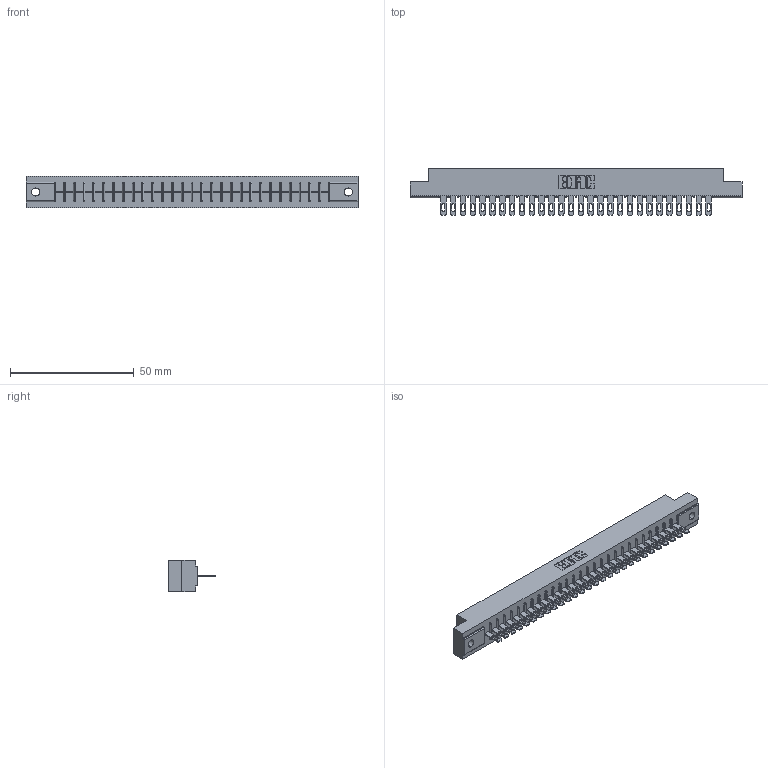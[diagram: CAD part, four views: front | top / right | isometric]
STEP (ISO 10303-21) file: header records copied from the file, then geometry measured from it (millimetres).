
FILE_DESCRIPTION (( 'STEP AP203' ), '1' );
FILE_NAME ('316-028-400-102.STEP', '2020-09-22T23:15:28', ( '' ), ( '' ), 'SwSTEP 2.0', 'SolidWorks 2020', '' );
FILE_SCHEMA (( 'CONFIG_CONTROL_DESIGN' ));
Length unit declared in the file: inch
Products named in the file (3): 316-028-400-102; 306 Part_.128 Dia; 306-290-001_100
Assembly tree (29 placements, depth 2):
  316-028-400-102
    306 Part_.128 Dia
    306-290-001_100  x28
Bounding box: 133.96 x 18.87 x 12.7 mm (x, y, z)
Volume: 14744.6 mm3; surface area: 15188.9 mm2
Topology: 29 solids, 29 shells, 2244 faces, 6336 edges, 4072 vertices
Faces by surface type: plane 1468, cylinder 664, sphere 112
Entity records: 28091 total; most frequent: CARTESIAN_POINT 4715, ORIENTED_EDGE 4672, DIRECTION 4652, EDGE_CURVE 2336, VECTOR 1818, LINE 1818, VERTEX_POINT 1480, AXIS2_PLACEMENT_3D 1417
